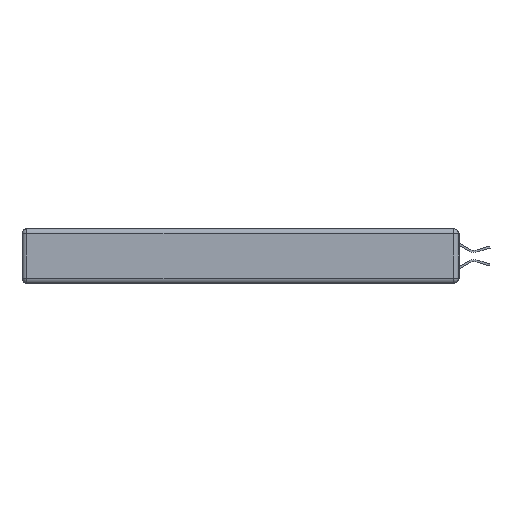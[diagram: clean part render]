
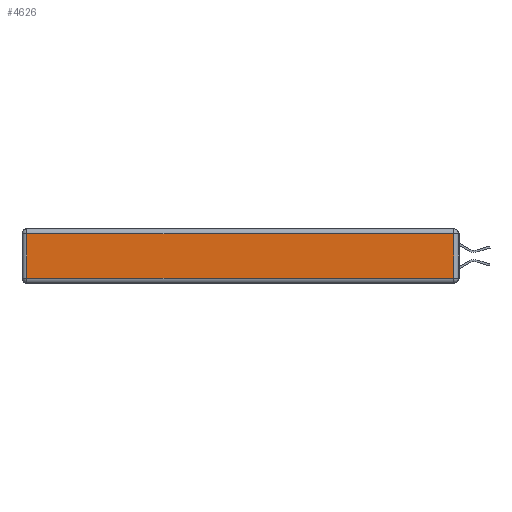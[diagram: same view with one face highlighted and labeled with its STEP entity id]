
A CAD part, left-side view. The second image highlights one B-rep face of the part: STEP entity #4626.
In plain terms, the highlighted planar face has unit normal (-1, 0, 0).
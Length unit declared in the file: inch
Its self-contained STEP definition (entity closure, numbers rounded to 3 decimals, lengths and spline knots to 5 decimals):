
#254 = VERTEX_POINT ( 'NONE', #20083 ) ;
#800 = DIRECTION ( 'NONE',  ( 0., -1., 0. ) ) ;
#1148 = DIRECTION ( 'NONE',  ( 0., 1., 0. ) ) ;
#1670 = VECTOR ( 'NONE', #2226, 39.37008 ) ;
#1835 = ORIENTED_EDGE ( 'NONE', *, *, #18747, .T. ) ;
#2005 = VERTEX_POINT ( 'NONE', #16900 ) ;
#2121 = EDGE_CURVE ( 'NONE', #254, #22805, #4253, .T. ) ;
#2194 = FACE_OUTER_BOUND ( 'NONE', #12829, .T. ) ;
#2226 = DIRECTION ( 'NONE',  ( 0., 0., 1. ) ) ;
#2667 = CARTESIAN_POINT ( 'NONE',  ( 0., 0., -0.343 ) ) ;
#4253 = LINE ( 'NONE', #11613, #16924 ) ;
#4551 = LINE ( 'NONE', #5910, #21790 ) ;
#4626 = ADVANCED_FACE ( 'NONE', ( #2194 ), #16851, .T. ) ;
#5873 = LINE ( 'NONE', #20803, #15728 ) ;
#5910 = CARTESIAN_POINT ( 'NONE',  ( 0., 2.72, -0.343 ) ) ;
#7442 = EDGE_CURVE ( 'NONE', #9340, #254, #4551, .T. ) ;
#8332 = EDGE_CURVE ( 'NONE', #22805, #2005, #22854, .T. ) ;
#9340 = VERTEX_POINT ( 'NONE', #14281 ) ;
#9826 = DIRECTION ( 'NONE',  ( 0., 0., 1. ) ) ;
#10707 = ORIENTED_EDGE ( 'NONE', *, *, #8332, .T. ) ;
#11080 = AXIS2_PLACEMENT_3D ( 'NONE', #2667, #13239, #9826 ) ;
#11186 = CARTESIAN_POINT ( 'NONE',  ( 0., 0.03, -0.343 ) ) ;
#11331 = DIRECTION ( 'NONE',  ( 0., 0., -1. ) ) ;
#11613 = CARTESIAN_POINT ( 'NONE',  ( 0., 0., -0.313 ) ) ;
#12829 = EDGE_LOOP ( 'NONE', ( #19947, #10707, #1835, #14292 ) ) ;
#13239 = DIRECTION ( 'NONE',  ( -1., 0., 0. ) ) ;
#14281 = CARTESIAN_POINT ( 'NONE',  ( 0., 2.72, -0.03 ) ) ;
#14292 = ORIENTED_EDGE ( 'NONE', *, *, #7442, .T. ) ;
#15728 = VECTOR ( 'NONE', #1148, 39.37008 ) ;
#16851 = PLANE ( 'NONE',  #11080 ) ;
#16900 = CARTESIAN_POINT ( 'NONE',  ( 0., 0.03, -0.03 ) ) ;
#16924 = VECTOR ( 'NONE', #800, 39.37008 ) ;
#18747 = EDGE_CURVE ( 'NONE', #2005, #9340, #5873, .T. ) ;
#19947 = ORIENTED_EDGE ( 'NONE', *, *, #2121, .T. ) ;
#20083 = CARTESIAN_POINT ( 'NONE',  ( 0., 2.72, -0.313 ) ) ;
#20803 = CARTESIAN_POINT ( 'NONE',  ( 0., 2.75, -0.03 ) ) ;
#20894 = CARTESIAN_POINT ( 'NONE',  ( 0., 0.03, -0.313 ) ) ;
#21790 = VECTOR ( 'NONE', #11331, 39.37008 ) ;
#22805 = VERTEX_POINT ( 'NONE', #20894 ) ;
#22854 = LINE ( 'NONE', #11186, #1670 ) ;
